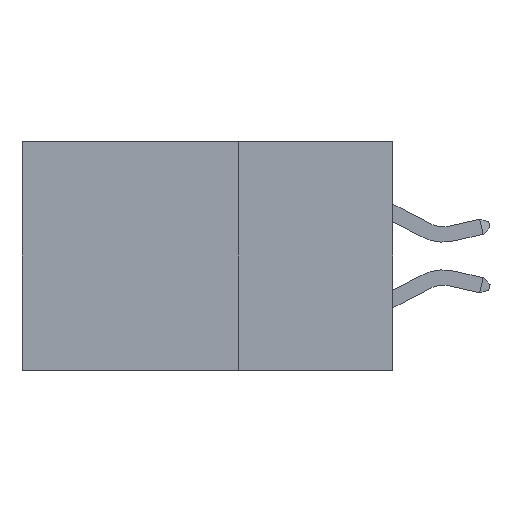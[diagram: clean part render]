
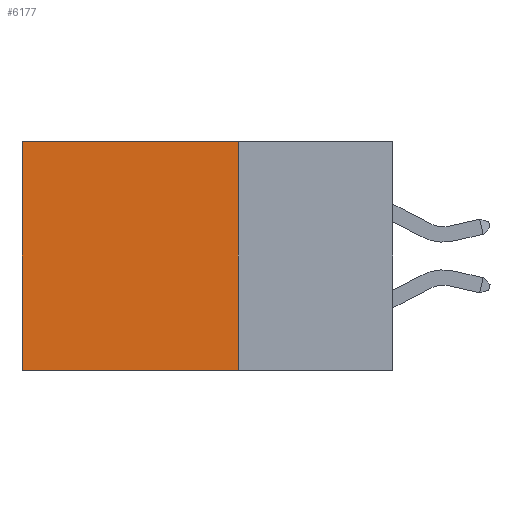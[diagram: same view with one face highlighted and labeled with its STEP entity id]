
A CAD part, left-side view. The second image highlights one B-rep face of the part: STEP entity #6177.
In plain terms, the highlighted planar face has unit normal (-1, 0, 0).
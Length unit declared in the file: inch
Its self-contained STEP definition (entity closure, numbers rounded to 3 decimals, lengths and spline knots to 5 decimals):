
#242 = VERTEX_POINT ( 'NONE', #21121 ) ;
#295 = VECTOR ( 'NONE', #6575, 39.37008 ) ;
#887 = EDGE_CURVE ( 'NONE', #242, #16388, #25027, .T. ) ;
#2462 = DIRECTION ( 'NONE',  ( 0., 1., 0. ) ) ;
#3452 = CARTESIAN_POINT ( 'NONE',  ( 0.2875, 0.6, -0.37 ) ) ;
#4075 = VECTOR ( 'NONE', #2462, 39.37008 ) ;
#6177 = ADVANCED_FACE ( 'NONE', ( #25698 ), #24905, .F. ) ;
#6575 = DIRECTION ( 'NONE',  ( 0., 0., -1. ) ) ;
#7374 = EDGE_LOOP ( 'NONE', ( #28285, #13714, #22508, #7548 ) ) ;
#7548 = ORIENTED_EDGE ( 'NONE', *, *, #28330, .T. ) ;
#8353 = VECTOR ( 'NONE', #19938, 39.37008 ) ;
#8528 = CARTESIAN_POINT ( 'NONE',  ( 0.2875, 0.25, 0. ) ) ;
#12245 = CARTESIAN_POINT ( 'NONE',  ( 0.2875, 0.25, 0. ) ) ;
#12501 = LINE ( 'NONE', #13933, #295 ) ;
#13328 = VERTEX_POINT ( 'NONE', #24981 ) ;
#13714 = ORIENTED_EDGE ( 'NONE', *, *, #887, .F. ) ;
#13933 = CARTESIAN_POINT ( 'NONE',  ( 0.2875, 0.6, 0. ) ) ;
#15404 = CARTESIAN_POINT ( 'NONE',  ( 0.2875, 0.25, 0. ) ) ;
#15448 = EDGE_CURVE ( 'NONE', #24471, #242, #23569, .T. ) ;
#15517 = DIRECTION ( 'NONE',  ( 0., 0., -1. ) ) ;
#16388 = VERTEX_POINT ( 'NONE', #3452 ) ;
#17213 = VECTOR ( 'NONE', #15517, 39.37008 ) ;
#19938 = DIRECTION ( 'NONE',  ( 0., 1., 0. ) ) ;
#21121 = CARTESIAN_POINT ( 'NONE',  ( 0.2875, 0.25, -0.37 ) ) ;
#22145 = CARTESIAN_POINT ( 'NONE',  ( 0.2875, 0.25, -0.37 ) ) ;
#22508 = ORIENTED_EDGE ( 'NONE', *, *, #15448, .F. ) ;
#22634 = DIRECTION ( 'NONE',  ( 1., 0., 0. ) ) ;
#22863 = EDGE_CURVE ( 'NONE', #13328, #16388, #12501, .T. ) ;
#23216 = AXIS2_PLACEMENT_3D ( 'NONE', #27295, #22634, #29857 ) ;
#23569 = LINE ( 'NONE', #15404, #17213 ) ;
#24471 = VERTEX_POINT ( 'NONE', #8528 ) ;
#24905 = PLANE ( 'NONE',  #23216 ) ;
#24981 = CARTESIAN_POINT ( 'NONE',  ( 0.2875, 0.6, 0. ) ) ;
#25027 = LINE ( 'NONE', #22145, #8353 ) ;
#25698 = FACE_OUTER_BOUND ( 'NONE', #7374, .T. ) ;
#27295 = CARTESIAN_POINT ( 'NONE',  ( 0.2875, 0.25, 0. ) ) ;
#28285 = ORIENTED_EDGE ( 'NONE', *, *, #22863, .T. ) ;
#28330 = EDGE_CURVE ( 'NONE', #24471, #13328, #29659, .T. ) ;
#29659 = LINE ( 'NONE', #12245, #4075 ) ;
#29857 = DIRECTION ( 'NONE',  ( 0., 0., -1. ) ) ;
